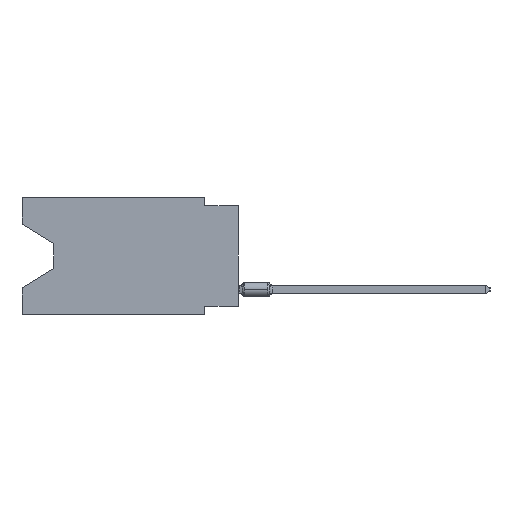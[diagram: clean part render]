
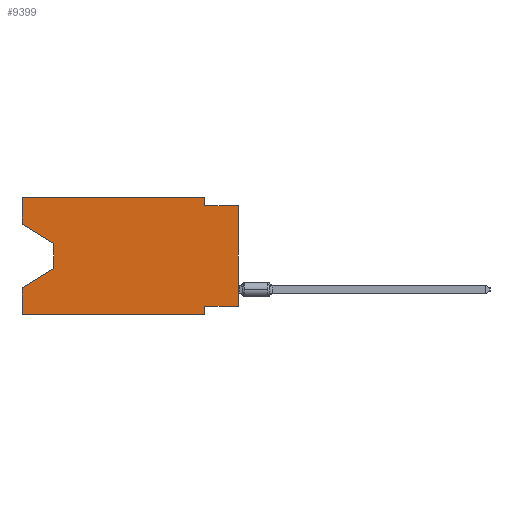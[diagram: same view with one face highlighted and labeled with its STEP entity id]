
A CAD part, left-side view. The second image highlights one B-rep face of the part: STEP entity #9399.
In plain terms, the highlighted planar face has unit normal (-1, 0, 0).
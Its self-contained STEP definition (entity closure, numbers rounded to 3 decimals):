
#61 = ORIENTED_EDGE ( 'NONE', *, *, #23655, .T. ) ;
#151 = EDGE_LOOP ( 'NONE', ( #37556, #19005, #1566, #10219, #61, #44934, #25488, #42705, #19192, #24881, #32752, #39079 ) ) ;
#566 = EDGE_CURVE ( 'NONE', #12460, #22932, #9980, .T. ) ;
#1437 = CARTESIAN_POINT ( 'NONE',  ( 0., 2.54, -0.635 ) ) ;
#1566 = ORIENTED_EDGE ( 'NONE', *, *, #35029, .T. ) ;
#2264 = VERTEX_POINT ( 'NONE', #15005 ) ;
#3660 = LINE ( 'NONE', #26479, #6818 ) ;
#4337 = EDGE_CURVE ( 'NONE', #46461, #41446, #7247, .T. ) ;
#4721 = VERTEX_POINT ( 'NONE', #26020 ) ;
#4885 = DIRECTION ( 'NONE',  ( 0., -1., 0. ) ) ;
#5441 = VERTEX_POINT ( 'NONE', #10821 ) ;
#6461 = CARTESIAN_POINT ( 'NONE',  ( 0., 0., 0. ) ) ;
#6783 = VERTEX_POINT ( 'NONE', #44822 ) ;
#6818 = VECTOR ( 'NONE', #4885, 1000. ) ;
#7247 = LINE ( 'NONE', #34022, #9997 ) ;
#7620 = CARTESIAN_POINT ( 'NONE',  ( 0., 2.54, 0. ) ) ;
#8016 = AXIS2_PLACEMENT_3D ( 'NONE', #28205, #9368, #14048 ) ;
#8453 = VECTOR ( 'NONE', #21546, 1000. ) ;
#9368 = DIRECTION ( 'NONE',  ( 1., 0., 0. ) ) ;
#9399 = ADVANCED_FACE ( 'NONE', ( #47317 ), #17539, .F. ) ;
#9980 = LINE ( 'NONE', #17428, #35989 ) ;
#9997 = VECTOR ( 'NONE', #21860, 1000. ) ;
#10219 = ORIENTED_EDGE ( 'NONE', *, *, #18662, .F. ) ;
#10821 = CARTESIAN_POINT ( 'NONE',  ( 0., 16.383, -2.038 ) ) ;
#10847 = EDGE_CURVE ( 'NONE', #34859, #36453, #41355, .T. ) ;
#11535 = VECTOR ( 'NONE', #38940, 1000. ) ;
#12444 = CARTESIAN_POINT ( 'NONE',  ( 0., 13.97, -5.385 ) ) ;
#12460 = VERTEX_POINT ( 'NONE', #42676 ) ;
#13317 = VECTOR ( 'NONE', #43304, 1000. ) ;
#13415 = DIRECTION ( 'NONE',  ( 0., 0., 1. ) ) ;
#14048 = DIRECTION ( 'NONE',  ( 0., 0., -1. ) ) ;
#14395 = EDGE_CURVE ( 'NONE', #5441, #6783, #22417, .T. ) ;
#15005 = CARTESIAN_POINT ( 'NONE',  ( 0., 0., -0.635 ) ) ;
#16309 = VECTOR ( 'NONE', #34076, 1000. ) ;
#17428 = CARTESIAN_POINT ( 'NONE',  ( 0., 13.97, -3.505 ) ) ;
#17539 = PLANE ( 'NONE',  #8016 ) ;
#18662 = EDGE_CURVE ( 'NONE', #37305, #4721, #28911, .T. ) ;
#18694 = CARTESIAN_POINT ( 'NONE',  ( 0., 16.383, 0. ) ) ;
#19005 = ORIENTED_EDGE ( 'NONE', *, *, #566, .T. ) ;
#19192 = ORIENTED_EDGE ( 'NONE', *, *, #38607, .F. ) ;
#19554 = EDGE_CURVE ( 'NONE', #41446, #28691, #46933, .T. ) ;
#20619 = LINE ( 'NONE', #6461, #36809 ) ;
#21546 = DIRECTION ( 'NONE',  ( 0., 0.855, -0.519 ) ) ;
#21674 = VECTOR ( 'NONE', #25190, 1000. ) ;
#21860 = DIRECTION ( 'NONE',  ( 0., 1., 0. ) ) ;
#22417 = LINE ( 'NONE', #18694, #16309 ) ;
#22741 = DIRECTION ( 'NONE',  ( 0., 0., -1. ) ) ;
#22932 = VERTEX_POINT ( 'NONE', #12444 ) ;
#22983 = EDGE_CURVE ( 'NONE', #46461, #2264, #20619, .T. ) ;
#23372 = EDGE_CURVE ( 'NONE', #5441, #12460, #45900, .T. ) ;
#23655 = EDGE_CURVE ( 'NONE', #37305, #28691, #3660, .T. ) ;
#24586 = DIRECTION ( 'NONE',  ( 0., 0., -1. ) ) ;
#24881 = ORIENTED_EDGE ( 'NONE', *, *, #10847, .F. ) ;
#25015 = LINE ( 'NONE', #43880, #8453 ) ;
#25190 = DIRECTION ( 'NONE',  ( 0., 0., 1. ) ) ;
#25488 = ORIENTED_EDGE ( 'NONE', *, *, #4337, .F. ) ;
#26020 = CARTESIAN_POINT ( 'NONE',  ( 0., 16.383, -6.852 ) ) ;
#26479 = CARTESIAN_POINT ( 'NONE',  ( 0., 16.383, -8.89 ) ) ;
#27296 = CARTESIAN_POINT ( 'NONE',  ( 0., 2.54, 0. ) ) ;
#28160 = CARTESIAN_POINT ( 'NONE',  ( 0., 0., -0.635 ) ) ;
#28185 = VECTOR ( 'NONE', #42392, 1000. ) ;
#28205 = CARTESIAN_POINT ( 'NONE',  ( 0., 16.383, 0. ) ) ;
#28609 = CARTESIAN_POINT ( 'NONE',  ( 0., 2.54, -8.255 ) ) ;
#28691 = VERTEX_POINT ( 'NONE', #30928 ) ;
#28899 = CARTESIAN_POINT ( 'NONE',  ( 0., 0., -8.255 ) ) ;
#28911 = LINE ( 'NONE', #44056, #21674 ) ;
#30928 = CARTESIAN_POINT ( 'NONE',  ( 0., 2.54, -8.89 ) ) ;
#31892 = LINE ( 'NONE', #28160, #13317 ) ;
#32752 = ORIENTED_EDGE ( 'NONE', *, *, #36291, .F. ) ;
#34022 = CARTESIAN_POINT ( 'NONE',  ( 0., 0., -8.255 ) ) ;
#34076 = DIRECTION ( 'NONE',  ( 0., 0., 1. ) ) ;
#34859 = VERTEX_POINT ( 'NONE', #27296 ) ;
#35029 = EDGE_CURVE ( 'NONE', #22932, #4721, #25015, .T. ) ;
#35978 = CARTESIAN_POINT ( 'NONE',  ( 0., 16.383, -8.89 ) ) ;
#35989 = VECTOR ( 'NONE', #43480, 1000. ) ;
#36291 = EDGE_CURVE ( 'NONE', #6783, #34859, #46123, .T. ) ;
#36453 = VERTEX_POINT ( 'NONE', #1437 ) ;
#36493 = VECTOR ( 'NONE', #24586, 1000. ) ;
#36809 = VECTOR ( 'NONE', #13415, 1000. ) ;
#37305 = VERTEX_POINT ( 'NONE', #35978 ) ;
#37556 = ORIENTED_EDGE ( 'NONE', *, *, #23372, .T. ) ;
#38607 = EDGE_CURVE ( 'NONE', #36453, #2264, #31892, .T. ) ;
#38940 = DIRECTION ( 'NONE',  ( 0., -0.855, -0.519 ) ) ;
#39079 = ORIENTED_EDGE ( 'NONE', *, *, #14395, .F. ) ;
#41355 = LINE ( 'NONE', #7620, #46920 ) ;
#41446 = VERTEX_POINT ( 'NONE', #28609 ) ;
#41664 = CARTESIAN_POINT ( 'NONE',  ( 0., 16.383, 0. ) ) ;
#42392 = DIRECTION ( 'NONE',  ( 0., -1., 0. ) ) ;
#42659 = CARTESIAN_POINT ( 'NONE',  ( 0., 16.383, -2.038 ) ) ;
#42676 = CARTESIAN_POINT ( 'NONE',  ( 0., 13.97, -3.505 ) ) ;
#42705 = ORIENTED_EDGE ( 'NONE', *, *, #22983, .T. ) ;
#43304 = DIRECTION ( 'NONE',  ( 0., -1., 0. ) ) ;
#43480 = DIRECTION ( 'NONE',  ( 0., 0., -1. ) ) ;
#43880 = CARTESIAN_POINT ( 'NONE',  ( 0., 13.97, -5.385 ) ) ;
#44056 = CARTESIAN_POINT ( 'NONE',  ( 0., 16.383, 0. ) ) ;
#44822 = CARTESIAN_POINT ( 'NONE',  ( 0., 16.383, 0. ) ) ;
#44934 = ORIENTED_EDGE ( 'NONE', *, *, #19554, .F. ) ;
#45900 = LINE ( 'NONE', #42659, #11535 ) ;
#46123 = LINE ( 'NONE', #41664, #28185 ) ;
#46461 = VERTEX_POINT ( 'NONE', #28899 ) ;
#46687 = CARTESIAN_POINT ( 'NONE',  ( 0., 2.54, -8.89 ) ) ;
#46920 = VECTOR ( 'NONE', #22741, 1000. ) ;
#46933 = LINE ( 'NONE', #46687, #36493 ) ;
#47317 = FACE_OUTER_BOUND ( 'NONE', #151, .T. ) ;
